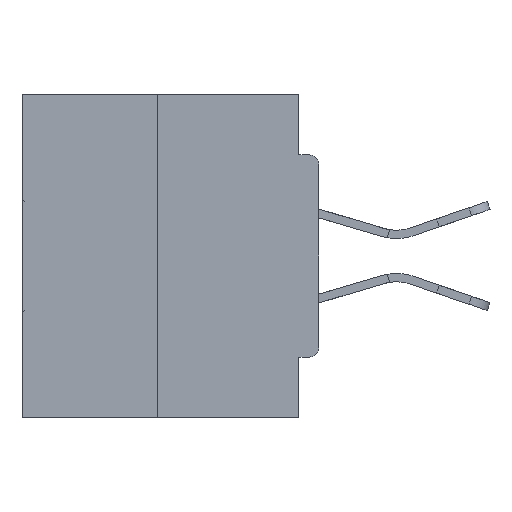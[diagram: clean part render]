
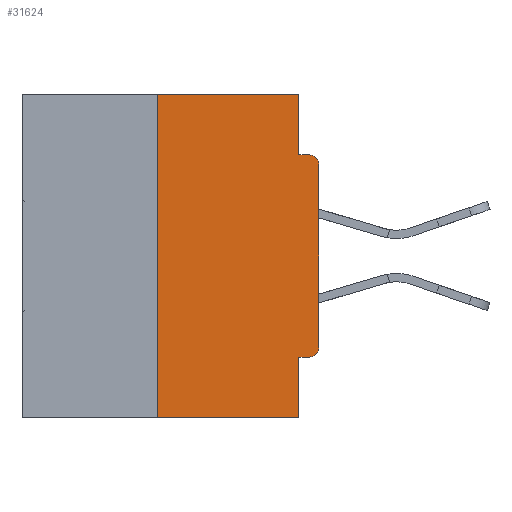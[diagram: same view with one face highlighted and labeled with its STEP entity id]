
A CAD part, left-side view. The second image highlights one B-rep face of the part: STEP entity #31624.
In plain terms, the highlighted planar face has unit normal (-1, 0, 0).
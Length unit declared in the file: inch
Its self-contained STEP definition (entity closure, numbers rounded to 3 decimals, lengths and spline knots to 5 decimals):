
#108 = AXIS2_PLACEMENT_3D ( 'NONE', #8735, #21805, #38702 ) ;
#372 = EDGE_CURVE ( 'NONE', #3840, #17564, #24974, .T. ) ;
#871 = FACE_OUTER_BOUND ( 'NONE', #25616, .T. ) ;
#2346 = LINE ( 'NONE', #12905, #22782 ) ;
#2654 = ORIENTED_EDGE ( 'NONE', *, *, #31717, .T. ) ;
#2775 = CARTESIAN_POINT ( 'NONE',  ( 0., 0., -0.1085 ) ) ;
#2870 = LINE ( 'NONE', #21855, #23836 ) ;
#3428 = LINE ( 'NONE', #22932, #23863 ) ;
#3507 = VECTOR ( 'NONE', #12165, 39.37008 ) ;
#3840 = VERTEX_POINT ( 'NONE', #4222 ) ;
#4222 = CARTESIAN_POINT ( 'NONE',  ( 0., 0.031, -0.4065 ) ) ;
#6425 = VERTEX_POINT ( 'NONE', #33768 ) ;
#6501 = CARTESIAN_POINT ( 'NONE',  ( 0., 0.031, -0.0935 ) ) ;
#6848 = EDGE_CURVE ( 'NONE', #17501, #28162, #12410, .T. ) ;
#6981 = VERTEX_POINT ( 'NONE', #42616 ) ;
#7765 = ORIENTED_EDGE ( 'NONE', *, *, #372, .F. ) ;
#7874 = CARTESIAN_POINT ( 'NONE',  ( 0., 0., -0.3915 ) ) ;
#8217 = CARTESIAN_POINT ( 'NONE',  ( 0., 0.25, 0. ) ) ;
#8735 = CARTESIAN_POINT ( 'NONE',  ( 0., 0.015, -0.3915 ) ) ;
#9760 = VERTEX_POINT ( 'NONE', #14307 ) ;
#11256 = DIRECTION ( 'NONE',  ( 0., -1., 0. ) ) ;
#12165 = DIRECTION ( 'NONE',  ( 0., 0., 1. ) ) ;
#12241 = CARTESIAN_POINT ( 'NONE',  ( 0., 0.031, 0. ) ) ;
#12410 = LINE ( 'NONE', #32467, #3507 ) ;
#12905 = CARTESIAN_POINT ( 'NONE',  ( 0., 0., -0.4065 ) ) ;
#13883 = ORIENTED_EDGE ( 'NONE', *, *, #32584, .F. ) ;
#14307 = CARTESIAN_POINT ( 'NONE',  ( 0., 0.25, 0. ) ) ;
#14559 = AXIS2_PLACEMENT_3D ( 'NONE', #18176, #31699, #14905 ) ;
#14905 = DIRECTION ( 'NONE',  ( 0., 0., -1. ) ) ;
#15254 = EDGE_CURVE ( 'NONE', #19899, #6425, #3428, .T. ) ;
#15409 = AXIS2_PLACEMENT_3D ( 'NONE', #17437, #27435, #24040 ) ;
#15605 = CARTESIAN_POINT ( 'NONE',  ( 0., 0.031, -0.5 ) ) ;
#15742 = CARTESIAN_POINT ( 'NONE',  ( 0., 0.015, -0.4065 ) ) ;
#16007 = LINE ( 'NONE', #38507, #33860 ) ;
#16204 = EDGE_CURVE ( 'NONE', #31784, #9760, #18814, .T. ) ;
#16529 = LINE ( 'NONE', #12241, #23891 ) ;
#17437 = CARTESIAN_POINT ( 'NONE',  ( 0., 0.46, 0. ) ) ;
#17501 = VERTEX_POINT ( 'NONE', #7874 ) ;
#17564 = VERTEX_POINT ( 'NONE', #15605 ) ;
#17567 = EDGE_CURVE ( 'NONE', #6981, #19899, #16529, .T. ) ;
#17832 = EDGE_CURVE ( 'NONE', #9760, #6981, #16007, .T. ) ;
#18176 = CARTESIAN_POINT ( 'NONE',  ( 0., 0.015, -0.1085 ) ) ;
#18814 = LINE ( 'NONE', #8217, #28222 ) ;
#18921 = ORIENTED_EDGE ( 'NONE', *, *, #16204, .F. ) ;
#19899 = VERTEX_POINT ( 'NONE', #6501 ) ;
#21767 = DIRECTION ( 'NONE',  ( 0., 0., -1. ) ) ;
#21805 = DIRECTION ( 'NONE',  ( -1., 0., 0. ) ) ;
#21855 = CARTESIAN_POINT ( 'NONE',  ( 0., 0.46, -0.5 ) ) ;
#22539 = DIRECTION ( 'NONE',  ( 0., 0., -1. ) ) ;
#22782 = VECTOR ( 'NONE', #33183, 39.37008 ) ;
#22932 = CARTESIAN_POINT ( 'NONE',  ( 0., 0., -0.0935 ) ) ;
#23392 = VECTOR ( 'NONE', #21767, 39.37008 ) ;
#23836 = VECTOR ( 'NONE', #11256, 39.37008 ) ;
#23863 = VECTOR ( 'NONE', #33071, 39.37008 ) ;
#23891 = VECTOR ( 'NONE', #22539, 39.37008 ) ;
#24040 = DIRECTION ( 'NONE',  ( 0., 0., -1. ) ) ;
#24187 = PLANE ( 'NONE',  #15409 ) ;
#24898 = EDGE_CURVE ( 'NONE', #27622, #17501, #38683, .T. ) ;
#24964 = ORIENTED_EDGE ( 'NONE', *, *, #17567, .F. ) ;
#24974 = LINE ( 'NONE', #31452, #23392 ) ;
#25616 = EDGE_LOOP ( 'NONE', ( #27240, #18921, #42382, #7765, #13883, #43236, #40438, #2654, #38228, #24964 ) ) ;
#27240 = ORIENTED_EDGE ( 'NONE', *, *, #17832, .F. ) ;
#27435 = DIRECTION ( 'NONE',  ( 1., 0., 0. ) ) ;
#27622 = VERTEX_POINT ( 'NONE', #15742 ) ;
#28162 = VERTEX_POINT ( 'NONE', #2775 ) ;
#28222 = VECTOR ( 'NONE', #28445, 39.37008 ) ;
#28445 = DIRECTION ( 'NONE',  ( 0., 0., 1. ) ) ;
#31452 = CARTESIAN_POINT ( 'NONE',  ( 0., 0.031, -0.5 ) ) ;
#31624 = ADVANCED_FACE ( 'NONE', ( #871 ), #24187, .F. ) ;
#31699 = DIRECTION ( 'NONE',  ( -1., 0., 0. ) ) ;
#31717 = EDGE_CURVE ( 'NONE', #28162, #6425, #39671, .T. ) ;
#31784 = VERTEX_POINT ( 'NONE', #34610 ) ;
#32467 = CARTESIAN_POINT ( 'NONE',  ( 0., 0., 0. ) ) ;
#32584 = EDGE_CURVE ( 'NONE', #27622, #3840, #2346, .T. ) ;
#33071 = DIRECTION ( 'NONE',  ( 0., -1., 0. ) ) ;
#33183 = DIRECTION ( 'NONE',  ( 0., 1., 0. ) ) ;
#33768 = CARTESIAN_POINT ( 'NONE',  ( 0., 0.015, -0.0935 ) ) ;
#33860 = VECTOR ( 'NONE', #34804, 39.37008 ) ;
#34610 = CARTESIAN_POINT ( 'NONE',  ( 0., 0.25, -0.5 ) ) ;
#34804 = DIRECTION ( 'NONE',  ( 0., -1., 0. ) ) ;
#38228 = ORIENTED_EDGE ( 'NONE', *, *, #15254, .F. ) ;
#38507 = CARTESIAN_POINT ( 'NONE',  ( 0., 0.46, 0. ) ) ;
#38683 = CIRCLE ( 'NONE', #108, 0.015 ) ;
#38702 = DIRECTION ( 'NONE',  ( 0., 0., -1. ) ) ;
#38963 = EDGE_CURVE ( 'NONE', #31784, #17564, #2870, .T. ) ;
#39671 = CIRCLE ( 'NONE', #14559, 0.015 ) ;
#40438 = ORIENTED_EDGE ( 'NONE', *, *, #6848, .T. ) ;
#42382 = ORIENTED_EDGE ( 'NONE', *, *, #38963, .T. ) ;
#42616 = CARTESIAN_POINT ( 'NONE',  ( 0., 0.031, 0. ) ) ;
#43236 = ORIENTED_EDGE ( 'NONE', *, *, #24898, .T. ) ;
